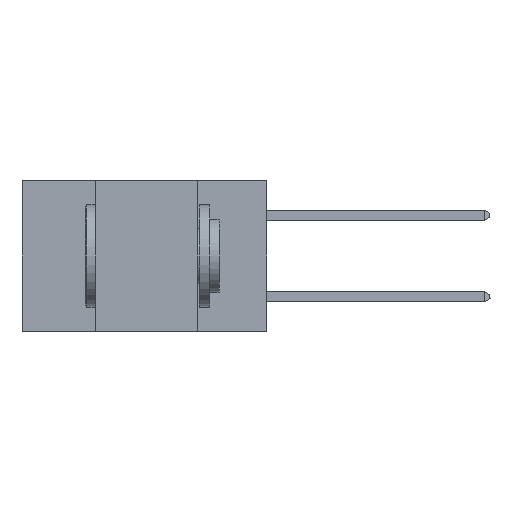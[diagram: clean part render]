
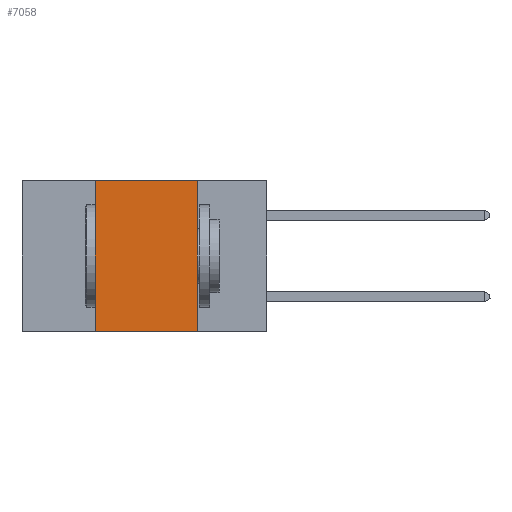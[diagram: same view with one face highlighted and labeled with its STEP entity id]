
A CAD part, left-side view. The second image highlights one B-rep face of the part: STEP entity #7058.
In plain terms, the highlighted planar face has unit normal (-1, 0, 0).
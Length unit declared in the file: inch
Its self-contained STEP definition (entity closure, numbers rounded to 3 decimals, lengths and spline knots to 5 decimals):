
#340 = EDGE_CURVE ( 'NONE', #831, #6806, #12162, .T. ) ;
#545 = CARTESIAN_POINT ( 'NONE',  ( 0., 0.42, 0. ) ) ;
#831 = VERTEX_POINT ( 'NONE', #19799 ) ;
#1137 = VECTOR ( 'NONE', #23442, 39.37008 ) ;
#3138 = AXIS2_PLACEMENT_3D ( 'NONE', #5744, #22187, #9887 ) ;
#3320 = CARTESIAN_POINT ( 'NONE',  ( 0., 0.6, 0. ) ) ;
#4019 = LINE ( 'NONE', #11533, #15015 ) ;
#4376 = LINE ( 'NONE', #3320, #9224 ) ;
#4530 = ORIENTED_EDGE ( 'NONE', *, *, #340, .T. ) ;
#4536 = EDGE_LOOP ( 'NONE', ( #18399, #8089, #14227, #4530 ) ) ;
#4626 = VECTOR ( 'NONE', #8928, 39.37008 ) ;
#5397 = FACE_OUTER_BOUND ( 'NONE', #4536, .T. ) ;
#5744 = CARTESIAN_POINT ( 'NONE',  ( 0., 0.6, 0. ) ) ;
#6806 = VERTEX_POINT ( 'NONE', #17384 ) ;
#7058 = ADVANCED_FACE ( 'NONE', ( #5397 ), #7816, .F. ) ;
#7816 = PLANE ( 'NONE',  #3138 ) ;
#8089 = ORIENTED_EDGE ( 'NONE', *, *, #12102, .F. ) ;
#8782 = VERTEX_POINT ( 'NONE', #545 ) ;
#8928 = DIRECTION ( 'NONE',  ( 0., 0., 1. ) ) ;
#9224 = VECTOR ( 'NONE', #15710, 39.37008 ) ;
#9781 = VERTEX_POINT ( 'NONE', #22689 ) ;
#9887 = DIRECTION ( 'NONE',  ( 0., 0., -1. ) ) ;
#11533 = CARTESIAN_POINT ( 'NONE',  ( 0., 0.17, 0. ) ) ;
#12102 = EDGE_CURVE ( 'NONE', #8782, #9781, #4376, .T. ) ;
#12162 = LINE ( 'NONE', #17069, #1137 ) ;
#12325 = EDGE_CURVE ( 'NONE', #9781, #6806, #4019, .T. ) ;
#14227 = ORIENTED_EDGE ( 'NONE', *, *, #21105, .F. ) ;
#15015 = VECTOR ( 'NONE', #23894, 39.37008 ) ;
#15710 = DIRECTION ( 'NONE',  ( 0., -1., 0. ) ) ;
#17069 = CARTESIAN_POINT ( 'NONE',  ( 0., 0.6, -0.37 ) ) ;
#17384 = CARTESIAN_POINT ( 'NONE',  ( 0., 0.17, -0.37 ) ) ;
#18399 = ORIENTED_EDGE ( 'NONE', *, *, #12325, .F. ) ;
#19799 = CARTESIAN_POINT ( 'NONE',  ( 0., 0.42, -0.37 ) ) ;
#20401 = LINE ( 'NONE', #21222, #4626 ) ;
#21105 = EDGE_CURVE ( 'NONE', #831, #8782, #20401, .T. ) ;
#21222 = CARTESIAN_POINT ( 'NONE',  ( 0., 0.42, 0. ) ) ;
#22187 = DIRECTION ( 'NONE',  ( 1., 0., 0. ) ) ;
#22689 = CARTESIAN_POINT ( 'NONE',  ( 0., 0.17, 0. ) ) ;
#23442 = DIRECTION ( 'NONE',  ( 0., -1., 0. ) ) ;
#23894 = DIRECTION ( 'NONE',  ( 0., 0., -1. ) ) ;
